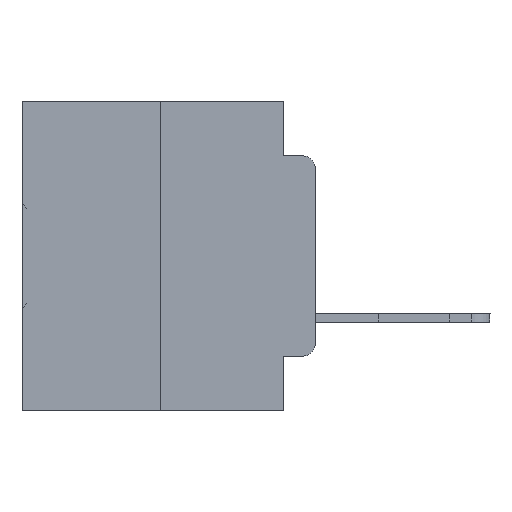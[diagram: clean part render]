
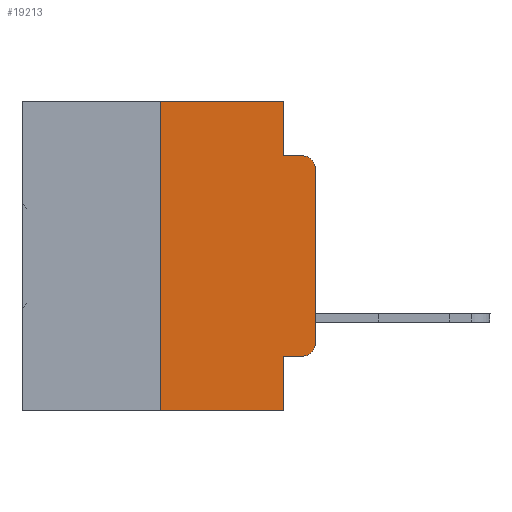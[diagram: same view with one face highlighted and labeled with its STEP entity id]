
A CAD part, left-side view. The second image highlights one B-rep face of the part: STEP entity #19213.
In plain terms, the highlighted planar face has unit normal (-1, 0, 0).
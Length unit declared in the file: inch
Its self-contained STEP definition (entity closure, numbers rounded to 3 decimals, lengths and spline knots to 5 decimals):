
#546 = LINE ( 'NONE', #1755, #15251 ) ;
#1155 = EDGE_CURVE ( 'NONE', #22905, #15945, #8517, .T. ) ;
#1755 = CARTESIAN_POINT ( 'NONE',  ( 0., 0.051, 0. ) ) ;
#2050 = EDGE_CURVE ( 'NONE', #28697, #15776, #19448, .T. ) ;
#2158 = AXIS2_PLACEMENT_3D ( 'NONE', #15818, #18455, #13107 ) ;
#5037 = VERTEX_POINT ( 'NONE', #13209 ) ;
#5154 = CARTESIAN_POINT ( 'NONE',  ( 0., 0.051, -0.5 ) ) ;
#5303 = VECTOR ( 'NONE', #29338, 39.37008 ) ;
#5872 = LINE ( 'NONE', #22852, #8311 ) ;
#6467 = ORIENTED_EDGE ( 'NONE', *, *, #26591, .F. ) ;
#6849 = VERTEX_POINT ( 'NONE', #11785 ) ;
#6886 = CIRCLE ( 'NONE', #23210, 0.02 ) ;
#6943 = CARTESIAN_POINT ( 'NONE',  ( 0., 0.051, -0.4115 ) ) ;
#7121 = DIRECTION ( 'NONE',  ( 0., 0., -1. ) ) ;
#7260 = EDGE_CURVE ( 'NONE', #20750, #22905, #23087, .T. ) ;
#7531 = ORIENTED_EDGE ( 'NONE', *, *, #26541, .F. ) ;
#7813 = ORIENTED_EDGE ( 'NONE', *, *, #8314, .F. ) ;
#8022 = EDGE_CURVE ( 'NONE', #18518, #10707, #18515, .T. ) ;
#8311 = VECTOR ( 'NONE', #20993, 39.37008 ) ;
#8314 = EDGE_CURVE ( 'NONE', #6849, #15776, #546, .T. ) ;
#8517 = LINE ( 'NONE', #15953, #28552 ) ;
#9611 = DIRECTION ( 'NONE',  ( 0., 0., -1. ) ) ;
#9751 = DIRECTION ( 'NONE',  ( 0., 0., -1. ) ) ;
#9888 = DIRECTION ( 'NONE',  ( 0., -1., 0. ) ) ;
#10413 = VECTOR ( 'NONE', #26467, 39.37008 ) ;
#10707 = VERTEX_POINT ( 'NONE', #32920 ) ;
#11631 = CARTESIAN_POINT ( 'NONE',  ( 0., 0., -0.3915 ) ) ;
#11785 = CARTESIAN_POINT ( 'NONE',  ( 0., 0.051, -0.4115 ) ) ;
#11918 = FACE_OUTER_BOUND ( 'NONE', #26281, .T. ) ;
#12198 = LINE ( 'NONE', #27301, #5303 ) ;
#13107 = DIRECTION ( 'NONE',  ( 0., 0., -1. ) ) ;
#13209 = CARTESIAN_POINT ( 'NONE',  ( 0., 0.02, -0.0885 ) ) ;
#13652 = CARTESIAN_POINT ( 'NONE',  ( 0., 0.473, 0. ) ) ;
#13906 = ORIENTED_EDGE ( 'NONE', *, *, #7260, .T. ) ;
#14193 = EDGE_CURVE ( 'NONE', #6849, #20750, #26423, .T. ) ;
#14846 = DIRECTION ( 'NONE',  ( 1., 0., 0. ) ) ;
#15251 = VECTOR ( 'NONE', #7121, 39.37008 ) ;
#15776 = VERTEX_POINT ( 'NONE', #5154 ) ;
#15818 = CARTESIAN_POINT ( 'NONE',  ( 0., 0.02, -0.3915 ) ) ;
#15945 = VERTEX_POINT ( 'NONE', #32166 ) ;
#15953 = CARTESIAN_POINT ( 'NONE',  ( 0., 0., 0. ) ) ;
#16950 = EDGE_CURVE ( 'NONE', #28705, #5037, #5872, .T. ) ;
#17545 = CARTESIAN_POINT ( 'NONE',  ( 0., 0.02, -0.1085 ) ) ;
#17575 = PLANE ( 'NONE',  #22056 ) ;
#18455 = DIRECTION ( 'NONE',  ( -1., 0., 0. ) ) ;
#18515 = LINE ( 'NONE', #13652, #10413 ) ;
#18518 = VERTEX_POINT ( 'NONE', #20052 ) ;
#19213 = ADVANCED_FACE ( 'NONE', ( #11918 ), #17575, .F. ) ;
#19448 = LINE ( 'NONE', #28222, #24736 ) ;
#20052 = CARTESIAN_POINT ( 'NONE',  ( 0., 0.25, 0. ) ) ;
#20750 = VERTEX_POINT ( 'NONE', #27685 ) ;
#20993 = DIRECTION ( 'NONE',  ( 0., -1., 0. ) ) ;
#21472 = EDGE_CURVE ( 'NONE', #15945, #5037, #6886, .T. ) ;
#22056 = AXIS2_PLACEMENT_3D ( 'NONE', #32996, #14846, #9751 ) ;
#22643 = DIRECTION ( 'NONE',  ( 0., -1., 0. ) ) ;
#22852 = CARTESIAN_POINT ( 'NONE',  ( 0., 0.051, -0.0885 ) ) ;
#22905 = VERTEX_POINT ( 'NONE', #11631 ) ;
#23087 = CIRCLE ( 'NONE', #2158, 0.02 ) ;
#23210 = AXIS2_PLACEMENT_3D ( 'NONE', #17545, #33187, #9611 ) ;
#23371 = ORIENTED_EDGE ( 'NONE', *, *, #21472, .T. ) ;
#24736 = VECTOR ( 'NONE', #9888, 39.37008 ) ;
#26129 = CARTESIAN_POINT ( 'NONE',  ( 0., 0.051, -0.0885 ) ) ;
#26281 = EDGE_LOOP ( 'NONE', ( #32326, #23371, #33646, #7531, #29066, #6467, #29317, #7813, #31053, #13906 ) ) ;
#26423 = LINE ( 'NONE', #6943, #30532 ) ;
#26467 = DIRECTION ( 'NONE',  ( 0., -1., 0. ) ) ;
#26541 = EDGE_CURVE ( 'NONE', #10707, #28705, #30580, .T. ) ;
#26591 = EDGE_CURVE ( 'NONE', #28697, #18518, #12198, .T. ) ;
#27301 = CARTESIAN_POINT ( 'NONE',  ( 0., 0.25, 0. ) ) ;
#27685 = CARTESIAN_POINT ( 'NONE',  ( 0., 0.02, -0.4115 ) ) ;
#28222 = CARTESIAN_POINT ( 'NONE',  ( 0., 0.473, -0.5 ) ) ;
#28552 = VECTOR ( 'NONE', #29207, 39.37008 ) ;
#28668 = CARTESIAN_POINT ( 'NONE',  ( 0., 0.25, -0.5 ) ) ;
#28697 = VERTEX_POINT ( 'NONE', #28668 ) ;
#28705 = VERTEX_POINT ( 'NONE', #26129 ) ;
#29066 = ORIENTED_EDGE ( 'NONE', *, *, #8022, .F. ) ;
#29207 = DIRECTION ( 'NONE',  ( 0., 0., 1. ) ) ;
#29317 = ORIENTED_EDGE ( 'NONE', *, *, #2050, .T. ) ;
#29338 = DIRECTION ( 'NONE',  ( 0., 0., 1. ) ) ;
#29799 = DIRECTION ( 'NONE',  ( 0., 0., -1. ) ) ;
#30532 = VECTOR ( 'NONE', #22643, 39.37008 ) ;
#30580 = LINE ( 'NONE', #32053, #33398 ) ;
#31053 = ORIENTED_EDGE ( 'NONE', *, *, #14193, .T. ) ;
#32053 = CARTESIAN_POINT ( 'NONE',  ( 0., 0.051, 0. ) ) ;
#32166 = CARTESIAN_POINT ( 'NONE',  ( 0., 0., -0.1085 ) ) ;
#32326 = ORIENTED_EDGE ( 'NONE', *, *, #1155, .T. ) ;
#32920 = CARTESIAN_POINT ( 'NONE',  ( 0., 0.051, 0. ) ) ;
#32996 = CARTESIAN_POINT ( 'NONE',  ( 0., 0.473, 0. ) ) ;
#33187 = DIRECTION ( 'NONE',  ( -1., 0., 0. ) ) ;
#33398 = VECTOR ( 'NONE', #29799, 39.37008 ) ;
#33646 = ORIENTED_EDGE ( 'NONE', *, *, #16950, .F. ) ;
